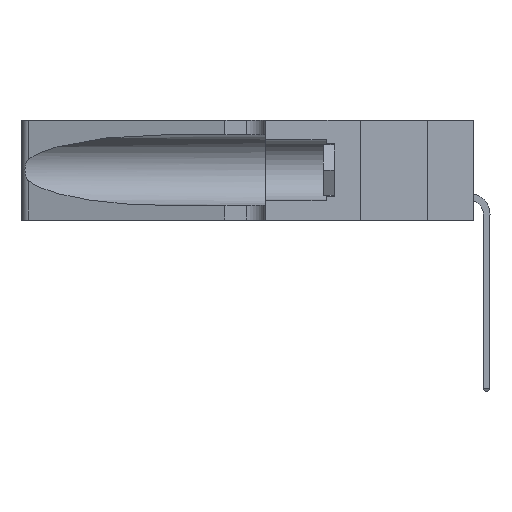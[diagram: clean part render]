
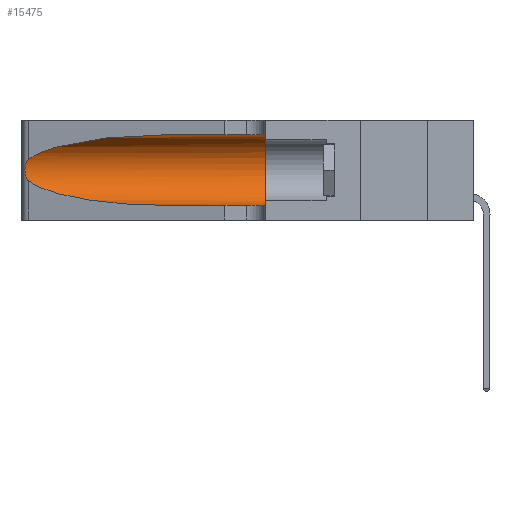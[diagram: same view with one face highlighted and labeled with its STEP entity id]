
A CAD part, left-side view. The second image highlights one B-rep face of the part: STEP entity #15475.
In plain terms, the highlighted cylindrical face has radius 3.308 mm (diameter 6.617 mm), a partial arc.
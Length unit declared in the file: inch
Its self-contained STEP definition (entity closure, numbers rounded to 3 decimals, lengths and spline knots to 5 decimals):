
#652 = CARTESIAN_POINT ( 'NONE',  ( 0.25487, 1.22718, 0.22369 ) ) ;
#693 = EDGE_CURVE ( 'NONE', #9849, #4866, #11183, .T. ) ;
#1141 = EDGE_CURVE ( 'NONE', #14313, #4866, #8673, .T. ) ;
#1270 = CARTESIAN_POINT ( 'NONE',  ( 0.18966, 0.96281, 0.05475 ) ) ;
#1876 = VERTEX_POINT ( 'NONE', #6724 ) ;
#1974 =( BOUNDED_CURVE ( )  B_SPLINE_CURVE ( 3, ( #5368, #16940, #1270, #8405 ),
 .UNSPECIFIED., .F., .T. ) 
 B_SPLINE_CURVE_WITH_KNOTS ( ( 4, 4 ),
 ( 3.44316, 4.71239 ),
 .UNSPECIFIED. ) 
 CURVE ( )  GEOMETRIC_REPRESENTATION_ITEM ( )  RATIONAL_B_SPLINE_CURVE ( ( 1., 0.87, 0.87, 1. ) ) 
 REPRESENTATION_ITEM ( '' )  );
#2408 = EDGE_CURVE ( 'NONE', #1876, #9849, #1974, .T. ) ;
#3083 = CARTESIAN_POINT ( 'NONE',  ( 0.1305, 0.72297, 0.05475 ) ) ;
#3121 = CARTESIAN_POINT ( 'NONE',  ( 0.25854, 1.2359, 0.20912 ) ) ;
#3246 = CARTESIAN_POINT ( 'NONE',  ( 0.26017, 1.23833, 0.17102 ) ) ;
#3849 = DIRECTION ( 'NONE',  ( 0., 1., 0. ) ) ;
#3981 = CARTESIAN_POINT ( 'NONE',  ( 0.1305, 0.35, 0.185 ) ) ;
#4607 = CARTESIAN_POINT ( 'NONE',  ( 0.25787, 1.23484, 0.2124 ) ) ;
#4630 = FACE_OUTER_BOUND ( 'NONE', #9564, .T. ) ;
#4666 = CARTESIAN_POINT ( 'NONE',  ( 0.25487, 1.22718, 0.22369 ) ) ;
#4677 = CARTESIAN_POINT ( 'NONE',  ( 0.25856, 1.23593, 0.16098 ) ) ;
#4742 = CARTESIAN_POINT ( 'NONE',  ( 0.25555, 1.22993, 0.14849 ) ) ;
#4813 = CARTESIAN_POINT ( 'NONE',  ( 0.18966, 0.96281, 0.31525 ) ) ;
#4866 = VERTEX_POINT ( 'NONE', #17005 ) ;
#5282 = DIRECTION ( 'NONE',  ( 0., 0., 1. ) ) ;
#5368 = CARTESIAN_POINT ( 'NONE',  ( 0.25487, 1.22718, 0.14631 ) ) ;
#5448 = EDGE_CURVE ( 'NONE', #9651, #1876, #17168, .T. ) ;
#5667 = AXIS2_PLACEMENT_3D ( 'NONE', #3981, #3849, #5282 ) ;
#6412 = AXIS2_PLACEMENT_3D ( 'NONE', #8949, #9143, #14710 ) ;
#6724 = CARTESIAN_POINT ( 'NONE',  ( 0.25487, 1.22718, 0.14631 ) ) ;
#6756 = ORIENTED_EDGE ( 'NONE', *, *, #2408, .T. ) ;
#7384 = VECTOR ( 'NONE', #14963, 39.37008 ) ;
#8214 = CARTESIAN_POINT ( 'NONE',  ( 0.1305, 1.61858, 0.31525 ) ) ;
#8405 = CARTESIAN_POINT ( 'NONE',  ( 0.1305, 0.72297, 0.05475 ) ) ;
#8673 = CIRCLE ( 'NONE', #5667, 0.13025 ) ;
#8949 = CARTESIAN_POINT ( 'NONE',  ( 0.1305, 1.61858, 0.185 ) ) ;
#9143 = DIRECTION ( 'NONE',  ( 0., -1., 0. ) ) ;
#9171 = CARTESIAN_POINT ( 'NONE',  ( 0.1305, 0.72297, 0.31525 ) ) ;
#9335 = CARTESIAN_POINT ( 'NONE',  ( 0.1305, 1.61858, 0.05475 ) ) ;
#9564 = EDGE_LOOP ( 'NONE', ( #9899, #16654, #6756, #14068, #16021, #16896 ) ) ;
#9651 = VERTEX_POINT ( 'NONE', #4666 ) ;
#9849 = VERTEX_POINT ( 'NONE', #3083 ) ;
#9899 = ORIENTED_EDGE ( 'NONE', *, *, #17163, .T. ) ;
#9980 = CYLINDRICAL_SURFACE ( 'NONE', #6412, 0.13025 ) ;
#10287 = VECTOR ( 'NONE', #18221, 39.37008 ) ;
#10406 = CARTESIAN_POINT ( 'NONE',  ( 0.25789, 1.23486, 0.15765 ) ) ;
#10870 = EDGE_CURVE ( 'NONE', #12543, #14313, #18342, .T. ) ;
#11183 = LINE ( 'NONE', #9335, #7384 ) ;
#11714 = CARTESIAN_POINT ( 'NONE',  ( 0.25639, 1.23184, 0.21858 ) ) ;
#12240 =( BOUNDED_CURVE ( )  B_SPLINE_CURVE ( 3, ( #9171, #4813, #16217, #652 ),
 .UNSPECIFIED., .F., .F. ) 
 B_SPLINE_CURVE_WITH_KNOTS ( ( 4, 4 ),
 ( 1.5708, 2.84003 ),
 .UNSPECIFIED. ) 
 CURVE ( )  GEOMETRIC_REPRESENTATION_ITEM ( )  RATIONAL_B_SPLINE_CURVE ( ( 1., 0.87, 0.87, 1. ) ) 
 REPRESENTATION_ITEM ( '' )  );
#12543 = VERTEX_POINT ( 'NONE', #13305 ) ;
#13078 = CARTESIAN_POINT ( 'NONE',  ( 0.26018, 1.23835, 0.19895 ) ) ;
#13208 = CARTESIAN_POINT ( 'NONE',  ( 0.26075, 1.23896, 0.178 ) ) ;
#13305 = CARTESIAN_POINT ( 'NONE',  ( 0.1305, 0.72297, 0.31525 ) ) ;
#14068 = ORIENTED_EDGE ( 'NONE', *, *, #693, .T. ) ;
#14313 = VERTEX_POINT ( 'NONE', #15869 ) ;
#14586 = CARTESIAN_POINT ( 'NONE',  ( 0.26075, 1.23896, 0.19203 ) ) ;
#14710 = DIRECTION ( 'NONE',  ( 0., 0., -1. ) ) ;
#14963 = DIRECTION ( 'NONE',  ( 0., -1., 0. ) ) ;
#15475 = ADVANCED_FACE ( 'NONE', ( #4630 ), #9980, .F. ) ;
#15869 = CARTESIAN_POINT ( 'NONE',  ( 0.1305, 0.35, 0.31525 ) ) ;
#16021 = ORIENTED_EDGE ( 'NONE', *, *, #1141, .F. ) ;
#16217 = CARTESIAN_POINT ( 'NONE',  ( 0.2373, 1.15595, 0.28018 ) ) ;
#16318 = CARTESIAN_POINT ( 'NONE',  ( 0.25487, 1.22718, 0.14631 ) ) ;
#16654 = ORIENTED_EDGE ( 'NONE', *, *, #5448, .T. ) ;
#16896 = ORIENTED_EDGE ( 'NONE', *, *, #10870, .F. ) ;
#16940 = CARTESIAN_POINT ( 'NONE',  ( 0.2373, 1.15595, 0.08982 ) ) ;
#17005 = CARTESIAN_POINT ( 'NONE',  ( 0.1305, 0.35, 0.05475 ) ) ;
#17163 = EDGE_CURVE ( 'NONE', #12543, #9651, #12240, .T. ) ;
#17168 = B_SPLINE_CURVE_WITH_KNOTS ( 'NONE', 3,
 ( #17213, #17336, #11714, #4607, #3121, #13078, #14586, #13208, #3246, #4677, #10406, #17521, #4742, #16318 ),
 .UNSPECIFIED., .F., .F.,
 ( 4, 2, 2, 2, 2, 2, 4 ),
 ( 0., 0.00027, 0.00053, 0.00107, 0.0016, 0.00187, 0.00214 ),
 .UNSPECIFIED. ) ;
#17213 = CARTESIAN_POINT ( 'NONE',  ( 0.25487, 1.22718, 0.22369 ) ) ;
#17336 = CARTESIAN_POINT ( 'NONE',  ( 0.25555, 1.22994, 0.2215 ) ) ;
#17521 = CARTESIAN_POINT ( 'NONE',  ( 0.25639, 1.23186, 0.15144 ) ) ;
#18221 = DIRECTION ( 'NONE',  ( 0., -1., 0. ) ) ;
#18342 = LINE ( 'NONE', #8214, #10287 ) ;
